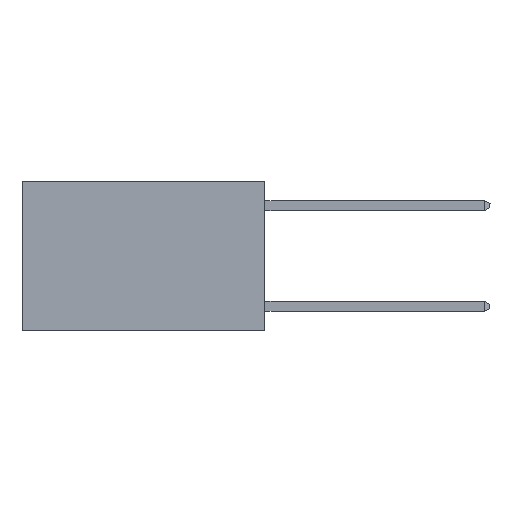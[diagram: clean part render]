
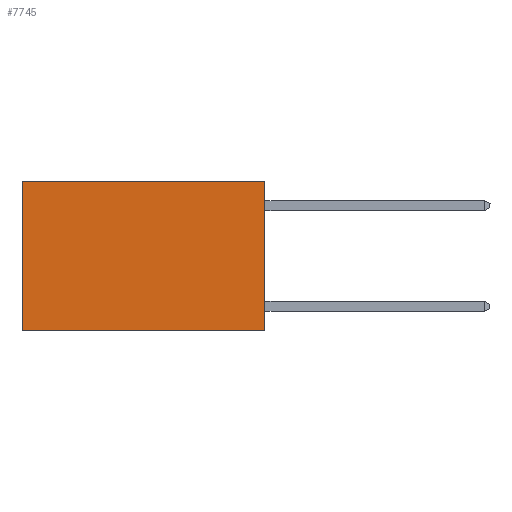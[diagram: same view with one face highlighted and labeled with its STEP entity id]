
A CAD part, left-side view. The second image highlights one B-rep face of the part: STEP entity #7745.
In plain terms, the highlighted planar face has unit normal (-1, 0, 0).
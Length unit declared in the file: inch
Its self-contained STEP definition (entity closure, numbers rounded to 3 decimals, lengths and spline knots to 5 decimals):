
#204 = CARTESIAN_POINT ( 'NONE',  ( 0.2625, 0., 0. ) ) ;
#1148 = CARTESIAN_POINT ( 'NONE',  ( 0.2625, 0., -0.37 ) ) ;
#1460 = VERTEX_POINT ( 'NONE', #12598 ) ;
#2860 = EDGE_LOOP ( 'NONE', ( #19004, #20517, #5921, #12204 ) ) ;
#3171 = VECTOR ( 'NONE', #13341, 39.37008 ) ;
#3849 = CARTESIAN_POINT ( 'NONE',  ( 0.2625, 0.6, 0. ) ) ;
#4119 = DIRECTION ( 'NONE',  ( 0., 1., 0. ) ) ;
#4178 = PLANE ( 'NONE',  #15965 ) ;
#4735 = DIRECTION ( 'NONE',  ( 0., 1., 0. ) ) ;
#5010 = VECTOR ( 'NONE', #4735, 39.37008 ) ;
#5183 = CARTESIAN_POINT ( 'NONE',  ( 0.2625, 0., -0.37 ) ) ;
#5712 = EDGE_CURVE ( 'NONE', #9715, #10963, #19069, .T. ) ;
#5921 = ORIENTED_EDGE ( 'NONE', *, *, #14766, .F. ) ;
#7065 = DIRECTION ( 'NONE',  ( 0., 0., -1. ) ) ;
#7378 = CARTESIAN_POINT ( 'NONE',  ( 0.2625, 0., 0. ) ) ;
#7424 = LINE ( 'NONE', #1148, #20231 ) ;
#7745 = ADVANCED_FACE ( 'NONE', ( #12265 ), #4178, .F. ) ;
#9715 = VERTEX_POINT ( 'NONE', #11184 ) ;
#9973 = LINE ( 'NONE', #204, #19849 ) ;
#10963 = VERTEX_POINT ( 'NONE', #3849 ) ;
#11032 = CARTESIAN_POINT ( 'NONE',  ( 0.2625, 0., 0. ) ) ;
#11184 = CARTESIAN_POINT ( 'NONE',  ( 0.2625, 0., 0. ) ) ;
#11786 = EDGE_CURVE ( 'NONE', #10963, #1460, #19711, .T. ) ;
#12204 = ORIENTED_EDGE ( 'NONE', *, *, #5712, .T. ) ;
#12265 = FACE_OUTER_BOUND ( 'NONE', #2860, .T. ) ;
#12598 = CARTESIAN_POINT ( 'NONE',  ( 0.2625, 0.6, -0.37 ) ) ;
#13341 = DIRECTION ( 'NONE',  ( 0., 0., -1. ) ) ;
#14766 = EDGE_CURVE ( 'NONE', #9715, #20183, #9973, .T. ) ;
#15342 = DIRECTION ( 'NONE',  ( 1., 0., 0. ) ) ;
#15965 = AXIS2_PLACEMENT_3D ( 'NONE', #7378, #15342, #7065 ) ;
#16209 = EDGE_CURVE ( 'NONE', #20183, #1460, #7424, .T. ) ;
#16450 = DIRECTION ( 'NONE',  ( 0., 0., -1. ) ) ;
#18120 = CARTESIAN_POINT ( 'NONE',  ( 0.2625, 0.6, 0. ) ) ;
#19004 = ORIENTED_EDGE ( 'NONE', *, *, #11786, .T. ) ;
#19069 = LINE ( 'NONE', #11032, #5010 ) ;
#19711 = LINE ( 'NONE', #18120, #3171 ) ;
#19849 = VECTOR ( 'NONE', #16450, 39.37008 ) ;
#20183 = VERTEX_POINT ( 'NONE', #5183 ) ;
#20231 = VECTOR ( 'NONE', #4119, 39.37008 ) ;
#20517 = ORIENTED_EDGE ( 'NONE', *, *, #16209, .F. ) ;
